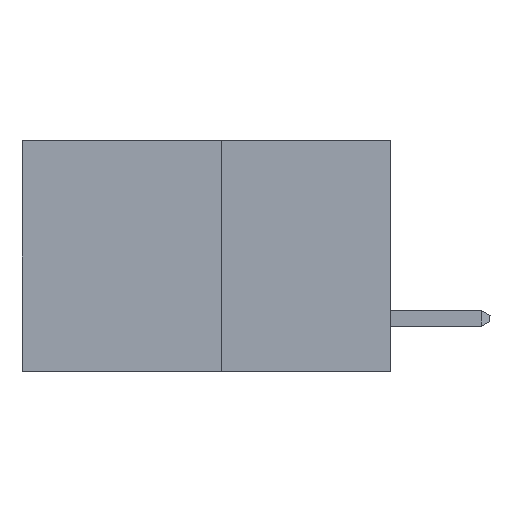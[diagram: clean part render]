
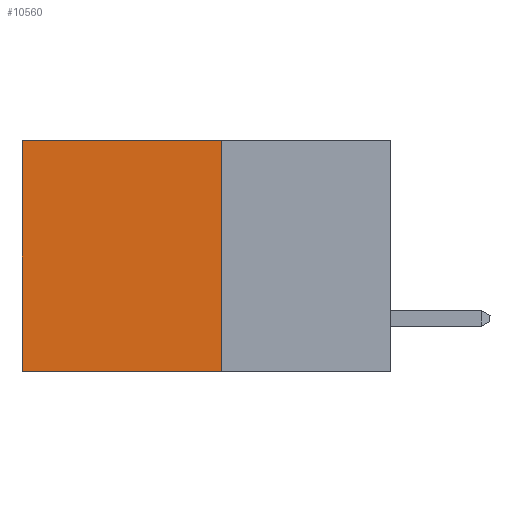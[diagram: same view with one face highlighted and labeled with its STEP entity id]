
A CAD part, left-side view. The second image highlights one B-rep face of the part: STEP entity #10560.
In plain terms, the highlighted planar face has unit normal (-1, 0, 0).
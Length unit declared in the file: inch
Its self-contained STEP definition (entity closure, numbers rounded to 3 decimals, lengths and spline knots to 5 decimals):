
#185 = DIRECTION ( 'NONE',  ( 0., 1., 0. ) ) ;
#985 = CARTESIAN_POINT ( 'NONE',  ( 0.277, 0.27, -0.37 ) ) ;
#1384 = ORIENTED_EDGE ( 'NONE', *, *, #2336, .T. ) ;
#1653 = AXIS2_PLACEMENT_3D ( 'NONE', #5296, #17510, #7056 ) ;
#2336 = EDGE_CURVE ( 'NONE', #13529, #17137, #3898, .T. ) ;
#3009 = LINE ( 'NONE', #4340, #21974 ) ;
#3898 = LINE ( 'NONE', #9479, #18304 ) ;
#4340 = CARTESIAN_POINT ( 'NONE',  ( 0.277, 0.27, -0.37 ) ) ;
#5294 = LINE ( 'NONE', #10584, #14644 ) ;
#5296 = CARTESIAN_POINT ( 'NONE',  ( 0.277, 0.27, -0.37 ) ) ;
#5526 = EDGE_LOOP ( 'NONE', ( #1384, #18411, #16777, #20553 ) ) ;
#5681 = CARTESIAN_POINT ( 'NONE',  ( 0.277, 0.59, 0. ) ) ;
#7056 = DIRECTION ( 'NONE',  ( 0., 0., -1. ) ) ;
#9479 = CARTESIAN_POINT ( 'NONE',  ( 0.277, 0.59, -0.37 ) ) ;
#9504 = CARTESIAN_POINT ( 'NONE',  ( 0.277, 0.27, 0. ) ) ;
#9717 = DIRECTION ( 'NONE',  ( 0., 0., -1. ) ) ;
#9941 = FACE_OUTER_BOUND ( 'NONE', #5526, .T. ) ;
#10560 = ADVANCED_FACE ( 'NONE', ( #9941 ), #14069, .F. ) ;
#10562 = EDGE_CURVE ( 'NONE', #20418, #13529, #5294, .T. ) ;
#10584 = CARTESIAN_POINT ( 'NONE',  ( 0.277, 0.27, 0. ) ) ;
#12308 = VERTEX_POINT ( 'NONE', #18170 ) ;
#12951 = VECTOR ( 'NONE', #20067, 39.37008 ) ;
#13529 = VERTEX_POINT ( 'NONE', #5681 ) ;
#14041 = LINE ( 'NONE', #985, #12951 ) ;
#14069 = PLANE ( 'NONE',  #1653 ) ;
#14644 = VECTOR ( 'NONE', #185, 39.37008 ) ;
#14806 = DIRECTION ( 'NONE',  ( 0., 0., -1. ) ) ;
#16777 = ORIENTED_EDGE ( 'NONE', *, *, #22394, .F. ) ;
#17137 = VERTEX_POINT ( 'NONE', #22115 ) ;
#17510 = DIRECTION ( 'NONE',  ( 1., 0., 0. ) ) ;
#18170 = CARTESIAN_POINT ( 'NONE',  ( 0.277, 0.27, -0.37 ) ) ;
#18304 = VECTOR ( 'NONE', #9717, 39.37008 ) ;
#18411 = ORIENTED_EDGE ( 'NONE', *, *, #19259, .F. ) ;
#19259 = EDGE_CURVE ( 'NONE', #12308, #17137, #14041, .T. ) ;
#20067 = DIRECTION ( 'NONE',  ( 0., 1., 0. ) ) ;
#20418 = VERTEX_POINT ( 'NONE', #9504 ) ;
#20553 = ORIENTED_EDGE ( 'NONE', *, *, #10562, .T. ) ;
#21974 = VECTOR ( 'NONE', #14806, 39.37008 ) ;
#22115 = CARTESIAN_POINT ( 'NONE',  ( 0.277, 0.59, -0.37 ) ) ;
#22394 = EDGE_CURVE ( 'NONE', #20418, #12308, #3009, .T. ) ;
